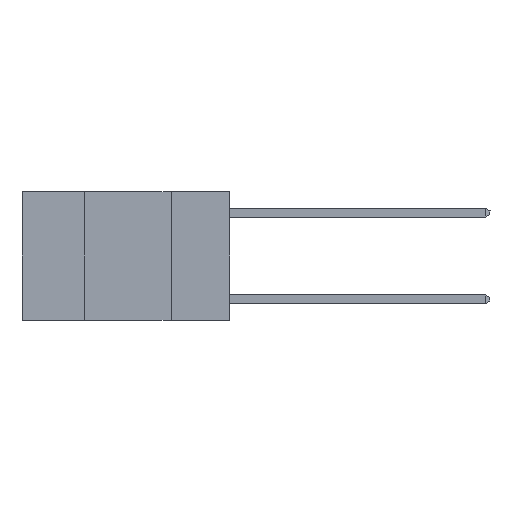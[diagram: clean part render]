
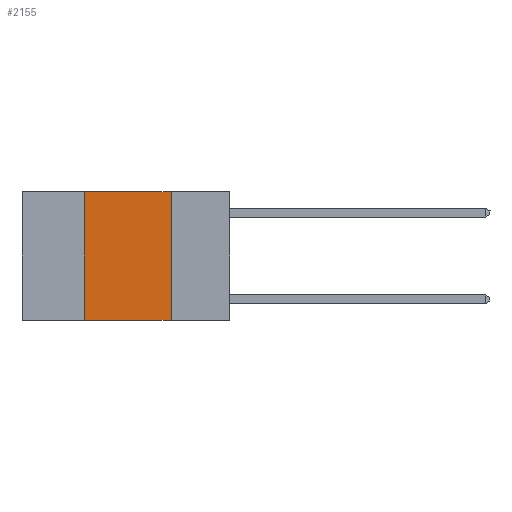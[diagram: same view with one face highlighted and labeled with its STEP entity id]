
A CAD part, left-side view. The second image highlights one B-rep face of the part: STEP entity #2155.
In plain terms, the highlighted planar face has unit normal (-1, 0, 0).
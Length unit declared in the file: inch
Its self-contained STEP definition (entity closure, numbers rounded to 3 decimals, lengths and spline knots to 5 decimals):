
#271 = EDGE_CURVE ( 'NONE', #313, #5110, #1148, .T. ) ;
#313 = VERTEX_POINT ( 'NONE', #5017 ) ;
#511 = VERTEX_POINT ( 'NONE', #9668 ) ;
#883 = VERTEX_POINT ( 'NONE', #8842 ) ;
#1148 = LINE ( 'NONE', #3289, #5223 ) ;
#1508 = CARTESIAN_POINT ( 'NONE',  ( 0., 0.17, -0.37 ) ) ;
#2079 = EDGE_CURVE ( 'NONE', #313, #883, #3501, .T. ) ;
#2155 = ADVANCED_FACE ( 'NONE', ( #8979 ), #7268, .F. ) ;
#2361 = CARTESIAN_POINT ( 'NONE',  ( 0., 0.6, 0. ) ) ;
#2988 = VECTOR ( 'NONE', #3083, 39.37008 ) ;
#3083 = DIRECTION ( 'NONE',  ( 0., 0., 1. ) ) ;
#3192 = DIRECTION ( 'NONE',  ( 1., 0., 0. ) ) ;
#3289 = CARTESIAN_POINT ( 'NONE',  ( 0., 0.6, -0.37 ) ) ;
#3356 = LINE ( 'NONE', #10103, #7675 ) ;
#3501 = LINE ( 'NONE', #3922, #2988 ) ;
#3624 = DIRECTION ( 'NONE',  ( 0., 0., -1. ) ) ;
#3655 = EDGE_LOOP ( 'NONE', ( #5825, #6819, #7077, #8454 ) ) ;
#3922 = CARTESIAN_POINT ( 'NONE',  ( 0., 0.42, 0. ) ) ;
#5017 = CARTESIAN_POINT ( 'NONE',  ( 0., 0.42, -0.37 ) ) ;
#5110 = VERTEX_POINT ( 'NONE', #1508 ) ;
#5223 = VECTOR ( 'NONE', #9609, 39.37008 ) ;
#5301 = DIRECTION ( 'NONE',  ( 0., -1., 0. ) ) ;
#5699 = VECTOR ( 'NONE', #5301, 39.37008 ) ;
#5825 = ORIENTED_EDGE ( 'NONE', *, *, #10254, .F. ) ;
#6819 = ORIENTED_EDGE ( 'NONE', *, *, #9576, .F. ) ;
#7077 = ORIENTED_EDGE ( 'NONE', *, *, #2079, .F. ) ;
#7268 = PLANE ( 'NONE',  #8098 ) ;
#7675 = VECTOR ( 'NONE', #3624, 39.37008 ) ;
#8098 = AXIS2_PLACEMENT_3D ( 'NONE', #2361, #3192, #8883 ) ;
#8454 = ORIENTED_EDGE ( 'NONE', *, *, #271, .T. ) ;
#8842 = CARTESIAN_POINT ( 'NONE',  ( 0., 0.42, 0. ) ) ;
#8883 = DIRECTION ( 'NONE',  ( 0., 0., -1. ) ) ;
#8979 = FACE_OUTER_BOUND ( 'NONE', #3655, .T. ) ;
#9576 = EDGE_CURVE ( 'NONE', #883, #511, #9727, .T. ) ;
#9609 = DIRECTION ( 'NONE',  ( 0., -1., 0. ) ) ;
#9668 = CARTESIAN_POINT ( 'NONE',  ( 0., 0.17, 0. ) ) ;
#9727 = LINE ( 'NONE', #10116, #5699 ) ;
#10103 = CARTESIAN_POINT ( 'NONE',  ( 0., 0.17, 0. ) ) ;
#10116 = CARTESIAN_POINT ( 'NONE',  ( 0., 0.6, 0. ) ) ;
#10254 = EDGE_CURVE ( 'NONE', #511, #5110, #3356, .T. ) ;
